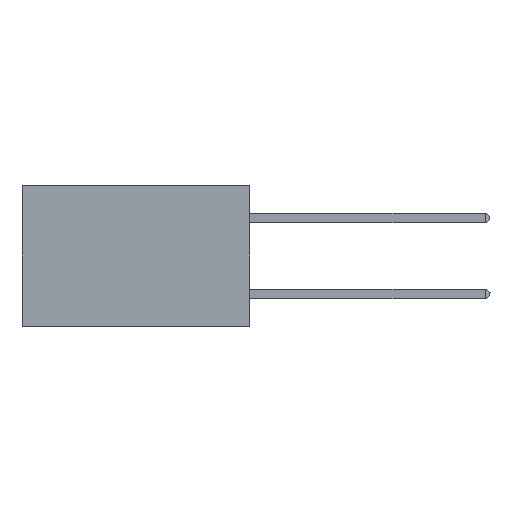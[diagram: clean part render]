
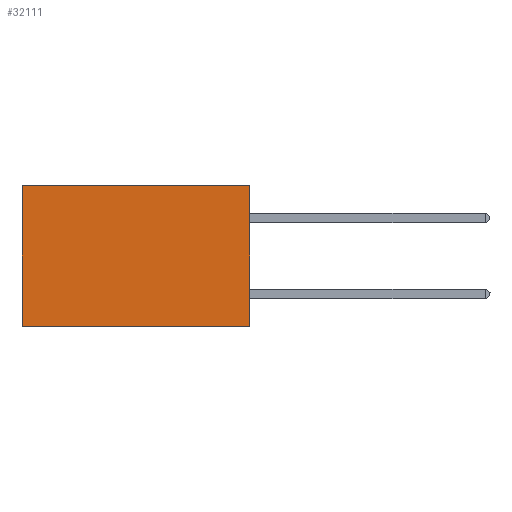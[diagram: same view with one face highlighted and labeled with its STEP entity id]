
A CAD part, left-side view. The second image highlights one B-rep face of the part: STEP entity #32111.
In plain terms, the highlighted planar face has unit normal (-1, 0, 0).
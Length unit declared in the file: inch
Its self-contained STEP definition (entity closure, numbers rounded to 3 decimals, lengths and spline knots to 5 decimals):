
#312 = VECTOR ( 'NONE', #34913, 39.37008 ) ;
#680 = CARTESIAN_POINT ( 'NONE',  ( 0.2875, 0.6, 0. ) ) ;
#923 = FACE_OUTER_BOUND ( 'NONE', #10843, .T. ) ;
#1417 = VECTOR ( 'NONE', #27271, 39.37008 ) ;
#1866 = VERTEX_POINT ( 'NONE', #40607 ) ;
#2476 = CARTESIAN_POINT ( 'NONE',  ( 0.2875, 0., -0.37 ) ) ;
#7242 = PLANE ( 'NONE',  #43534 ) ;
#7488 = LINE ( 'NONE', #33624, #31961 ) ;
#10777 = DIRECTION ( 'NONE',  ( 0., 0., -1. ) ) ;
#10843 = EDGE_LOOP ( 'NONE', ( #42502, #13684, #12991, #21029 ) ) ;
#11810 = LINE ( 'NONE', #34307, #312 ) ;
#12837 = DIRECTION ( 'NONE',  ( 0., 0., -1. ) ) ;
#12991 = ORIENTED_EDGE ( 'NONE', *, *, #15006, .F. ) ;
#13034 = VERTEX_POINT ( 'NONE', #2476 ) ;
#13684 = ORIENTED_EDGE ( 'NONE', *, *, #18988, .F. ) ;
#14647 = VERTEX_POINT ( 'NONE', #39325 ) ;
#15006 = EDGE_CURVE ( 'NONE', #14647, #13034, #37869, .T. ) ;
#18988 = EDGE_CURVE ( 'NONE', #13034, #1866, #28736, .T. ) ;
#19977 = EDGE_CURVE ( 'NONE', #34565, #1866, #7488, .T. ) ;
#21029 = ORIENTED_EDGE ( 'NONE', *, *, #27282, .T. ) ;
#24957 = VECTOR ( 'NONE', #36281, 39.37008 ) ;
#27271 = DIRECTION ( 'NONE',  ( 0., 0., -1. ) ) ;
#27282 = EDGE_CURVE ( 'NONE', #14647, #34565, #11810, .T. ) ;
#28736 = LINE ( 'NONE', #39799, #24957 ) ;
#31565 = DIRECTION ( 'NONE',  ( 1., 0., 0. ) ) ;
#31863 = CARTESIAN_POINT ( 'NONE',  ( 0.2875, 0., 0. ) ) ;
#31961 = VECTOR ( 'NONE', #12837, 39.37008 ) ;
#32111 = ADVANCED_FACE ( 'NONE', ( #923 ), #7242, .F. ) ;
#33624 = CARTESIAN_POINT ( 'NONE',  ( 0.2875, 0.6, 0. ) ) ;
#34307 = CARTESIAN_POINT ( 'NONE',  ( 0.2875, 0., 0. ) ) ;
#34565 = VERTEX_POINT ( 'NONE', #680 ) ;
#34913 = DIRECTION ( 'NONE',  ( 0., 1., 0. ) ) ;
#36281 = DIRECTION ( 'NONE',  ( 0., 1., 0. ) ) ;
#37869 = LINE ( 'NONE', #44907, #1417 ) ;
#39325 = CARTESIAN_POINT ( 'NONE',  ( 0.2875, 0., 0. ) ) ;
#39799 = CARTESIAN_POINT ( 'NONE',  ( 0.2875, 0., -0.37 ) ) ;
#40607 = CARTESIAN_POINT ( 'NONE',  ( 0.2875, 0.6, -0.37 ) ) ;
#42502 = ORIENTED_EDGE ( 'NONE', *, *, #19977, .T. ) ;
#43534 = AXIS2_PLACEMENT_3D ( 'NONE', #31863, #31565, #10777 ) ;
#44907 = CARTESIAN_POINT ( 'NONE',  ( 0.2875, 0., 0. ) ) ;
